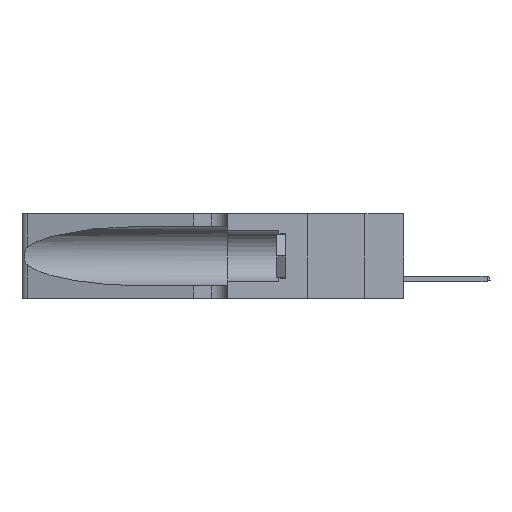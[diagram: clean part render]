
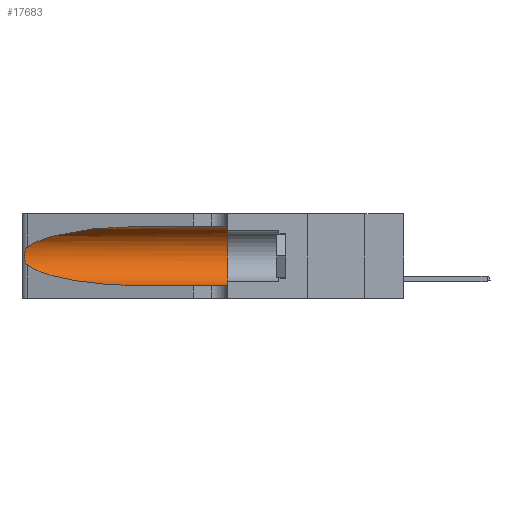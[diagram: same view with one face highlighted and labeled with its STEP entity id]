
A CAD part, left-side view. The second image highlights one B-rep face of the part: STEP entity #17683.
In plain terms, the highlighted cylindrical face has radius 3.308 mm (diameter 6.617 mm), a partial arc.
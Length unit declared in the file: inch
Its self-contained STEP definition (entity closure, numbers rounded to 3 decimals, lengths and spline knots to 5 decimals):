
#210 = VERTEX_POINT ( 'NONE', #13570 ) ;
#482 = CARTESIAN_POINT ( 'NONE',  ( 0.1305, 0.72297, 0.31525 ) ) ;
#805 = CARTESIAN_POINT ( 'NONE',  ( 0.1305, 0.72297, 0.31525 ) ) ;
#2129 = EDGE_CURVE ( 'NONE', #9981, #210, #3419, .T. ) ;
#3202 = VERTEX_POINT ( 'NONE', #13903 ) ;
#3417 = CARTESIAN_POINT ( 'NONE',  ( 0.2373, 1.15595, 0.28018 ) ) ;
#3419 = CIRCLE ( 'NONE', #15857, 0.13025 ) ;
#5237 = LINE ( 'NONE', #15457, #13876 ) ;
#5617 = CARTESIAN_POINT ( 'NONE',  ( 0.1305, 1.61858, 0.05475 ) ) ;
#6089 = VERTEX_POINT ( 'NONE', #805 ) ;
#6306 = EDGE_CURVE ( 'NONE', #34965, #3202, #9415, .T. ) ;
#8337 = CARTESIAN_POINT ( 'NONE',  ( 0.1305, 0.35, 0.31525 ) ) ;
#9415 =( BOUNDED_CURVE ( )  B_SPLINE_CURVE ( 3, ( #25461, #34758, #22773, #20081 ),
 .UNSPECIFIED., .F., .T. ) 
 B_SPLINE_CURVE_WITH_KNOTS ( ( 4, 4 ),
 ( 3.44316, 4.71239 ),
 .UNSPECIFIED. ) 
 CURVE ( )  GEOMETRIC_REPRESENTATION_ITEM ( )  RATIONAL_B_SPLINE_CURVE ( ( 1., 0.87, 0.87, 1. ) ) 
 REPRESENTATION_ITEM ( '' )  );
#9734 = CARTESIAN_POINT ( 'NONE',  ( 0.25856, 1.23593, 0.16098 ) ) ;
#9981 = VERTEX_POINT ( 'NONE', #8337 ) ;
#11161 = EDGE_CURVE ( 'NONE', #16977, #34965, #24740, .T. ) ;
#11295 = ORIENTED_EDGE ( 'NONE', *, *, #35871, .T. ) ;
#13570 = CARTESIAN_POINT ( 'NONE',  ( 0.1305, 0.35, 0.05475 ) ) ;
#13876 = VECTOR ( 'NONE', #15725, 39.37008 ) ;
#13903 = CARTESIAN_POINT ( 'NONE',  ( 0.1305, 0.72297, 0.05475 ) ) ;
#14656 =( BOUNDED_CURVE ( )  B_SPLINE_CURVE ( 3, ( #482, #20731, #3417, #26137 ),
 .UNSPECIFIED., .F., .F. ) 
 B_SPLINE_CURVE_WITH_KNOTS ( ( 4, 4 ),
 ( 1.5708, 2.84003 ),
 .UNSPECIFIED. ) 
 CURVE ( )  GEOMETRIC_REPRESENTATION_ITEM ( )  RATIONAL_B_SPLINE_CURVE ( ( 1., 0.87, 0.87, 1. ) ) 
 REPRESENTATION_ITEM ( '' )  );
#14661 = ORIENTED_EDGE ( 'NONE', *, *, #6306, .T. ) ;
#15457 = CARTESIAN_POINT ( 'NONE',  ( 0.1305, 1.61858, 0.31525 ) ) ;
#15725 = DIRECTION ( 'NONE',  ( 0., -1., 0. ) ) ;
#15857 = AXIS2_PLACEMENT_3D ( 'NONE', #31465, #36947, #23766 ) ;
#16917 = DIRECTION ( 'NONE',  ( 0., -1., 0. ) ) ;
#16977 = VERTEX_POINT ( 'NONE', #29982 ) ;
#17683 = ADVANCED_FACE ( 'NONE', ( #36513 ), #37433, .F. ) ;
#18052 = CARTESIAN_POINT ( 'NONE',  ( 0.25789, 1.23486, 0.15765 ) ) ;
#18300 = VECTOR ( 'NONE', #16917, 39.37008 ) ;
#18423 = CARTESIAN_POINT ( 'NONE',  ( 0.25555, 1.22993, 0.14849 ) ) ;
#18574 = AXIS2_PLACEMENT_3D ( 'NONE', #27956, #33547, #36863 ) ;
#19558 = ORIENTED_EDGE ( 'NONE', *, *, #11161, .T. ) ;
#20081 = CARTESIAN_POINT ( 'NONE',  ( 0.1305, 0.72297, 0.05475 ) ) ;
#20611 = ORIENTED_EDGE ( 'NONE', *, *, #35450, .F. ) ;
#20719 = CARTESIAN_POINT ( 'NONE',  ( 0.25487, 1.22718, 0.14631 ) ) ;
#20731 = CARTESIAN_POINT ( 'NONE',  ( 0.18966, 0.96281, 0.31525 ) ) ;
#20963 = CARTESIAN_POINT ( 'NONE',  ( 0.26075, 1.23896, 0.19203 ) ) ;
#21223 = CARTESIAN_POINT ( 'NONE',  ( 0.25639, 1.23186, 0.15144 ) ) ;
#21991 = LINE ( 'NONE', #5617, #18300 ) ;
#22773 = CARTESIAN_POINT ( 'NONE',  ( 0.18966, 0.96281, 0.05475 ) ) ;
#23051 = EDGE_CURVE ( 'NONE', #3202, #210, #21991, .T. ) ;
#23664 = CARTESIAN_POINT ( 'NONE',  ( 0.26017, 1.23833, 0.17102 ) ) ;
#23766 = DIRECTION ( 'NONE',  ( 0., 0., 1. ) ) ;
#24055 = CARTESIAN_POINT ( 'NONE',  ( 0.25787, 1.23484, 0.2124 ) ) ;
#24740 = B_SPLINE_CURVE_WITH_KNOTS ( 'NONE', 3,
 ( #26981, #29910, #35898, #24055, #26722, #26847, #20963, #27110, #23664, #9734, #18052, #21223, #18423, #20719 ),
 .UNSPECIFIED., .F., .F.,
 ( 4, 2, 2, 2, 2, 2, 4 ),
 ( 0., 0.00027, 0.00053, 0.00107, 0.0016, 0.00187, 0.00214 ),
 .UNSPECIFIED. ) ;
#25461 = CARTESIAN_POINT ( 'NONE',  ( 0.25487, 1.22718, 0.14631 ) ) ;
#26137 = CARTESIAN_POINT ( 'NONE',  ( 0.25487, 1.22718, 0.22369 ) ) ;
#26722 = CARTESIAN_POINT ( 'NONE',  ( 0.25854, 1.2359, 0.20912 ) ) ;
#26847 = CARTESIAN_POINT ( 'NONE',  ( 0.26018, 1.23835, 0.19895 ) ) ;
#26981 = CARTESIAN_POINT ( 'NONE',  ( 0.25487, 1.22718, 0.22369 ) ) ;
#27110 = CARTESIAN_POINT ( 'NONE',  ( 0.26075, 1.23896, 0.178 ) ) ;
#27253 = ORIENTED_EDGE ( 'NONE', *, *, #23051, .T. ) ;
#27956 = CARTESIAN_POINT ( 'NONE',  ( 0.1305, 1.61858, 0.185 ) ) ;
#29910 = CARTESIAN_POINT ( 'NONE',  ( 0.25555, 1.22994, 0.2215 ) ) ;
#29982 = CARTESIAN_POINT ( 'NONE',  ( 0.25487, 1.22718, 0.22369 ) ) ;
#31465 = CARTESIAN_POINT ( 'NONE',  ( 0.1305, 0.35, 0.185 ) ) ;
#33547 = DIRECTION ( 'NONE',  ( 0., -1., 0. ) ) ;
#34758 = CARTESIAN_POINT ( 'NONE',  ( 0.2373, 1.15595, 0.08982 ) ) ;
#34965 = VERTEX_POINT ( 'NONE', #35731 ) ;
#35450 = EDGE_CURVE ( 'NONE', #6089, #9981, #5237, .T. ) ;
#35731 = CARTESIAN_POINT ( 'NONE',  ( 0.25487, 1.22718, 0.14631 ) ) ;
#35744 = EDGE_LOOP ( 'NONE', ( #11295, #19558, #14661, #27253, #36377, #20611 ) ) ;
#35871 = EDGE_CURVE ( 'NONE', #6089, #16977, #14656, .T. ) ;
#35898 = CARTESIAN_POINT ( 'NONE',  ( 0.25639, 1.23184, 0.21858 ) ) ;
#36377 = ORIENTED_EDGE ( 'NONE', *, *, #2129, .F. ) ;
#36513 = FACE_OUTER_BOUND ( 'NONE', #35744, .T. ) ;
#36863 = DIRECTION ( 'NONE',  ( 0., 0., -1. ) ) ;
#36947 = DIRECTION ( 'NONE',  ( 0., 1., 0. ) ) ;
#37433 = CYLINDRICAL_SURFACE ( 'NONE', #18574, 0.13025 ) ;
